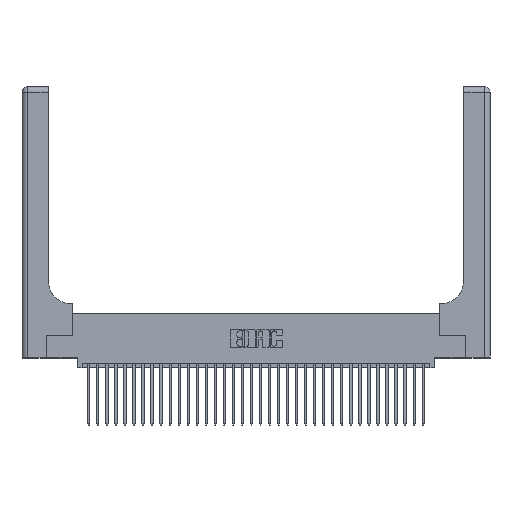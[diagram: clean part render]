
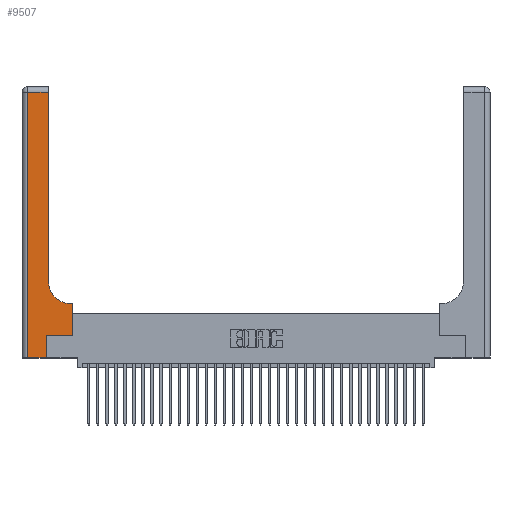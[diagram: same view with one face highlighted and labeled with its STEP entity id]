
A CAD part, top view. The second image highlights one B-rep face of the part: STEP entity #9507.
In plain terms, the highlighted planar face has unit normal (0, 0, 1).
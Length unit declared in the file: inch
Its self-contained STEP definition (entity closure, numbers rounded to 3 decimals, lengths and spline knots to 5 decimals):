
#9 = DIRECTION ( 'NONE',  ( 1., 0., 0. ) ) ;
#418 = VERTEX_POINT ( 'NONE', #31745 ) ;
#1889 = VECTOR ( 'NONE', #17187, 39.37008 ) ;
#2439 = CARTESIAN_POINT ( 'NONE',  ( 0., 0., 0.37 ) ) ;
#2482 = VECTOR ( 'NONE', #2788, 39.37008 ) ;
#2788 = DIRECTION ( 'NONE',  ( 0., 1., 0. ) ) ;
#2900 = DIRECTION ( 'NONE',  ( 0., -1., 0. ) ) ;
#3257 = CARTESIAN_POINT ( 'NONE',  ( 0.06, 3., 0.37 ) ) ;
#3908 = VERTEX_POINT ( 'NONE', #11138 ) ;
#4597 = DIRECTION ( 'NONE',  ( 0., 1., 0. ) ) ;
#4941 = EDGE_CURVE ( 'NONE', #12371, #28858, #16066, .T. ) ;
#6059 = ORIENTED_EDGE ( 'NONE', *, *, #20198, .T. ) ;
#6118 = ORIENTED_EDGE ( 'NONE', *, *, #13954, .T. ) ;
#6149 = VECTOR ( 'NONE', #17732, 39.37008 ) ;
#7418 = DIRECTION ( 'NONE',  ( 0., 0., -1. ) ) ;
#8572 = VERTEX_POINT ( 'NONE', #21850 ) ;
#9049 = VECTOR ( 'NONE', #17048, 39.37008 ) ;
#9247 = ORIENTED_EDGE ( 'NONE', *, *, #4941, .T. ) ;
#9507 = ADVANCED_FACE ( 'NONE', ( #16329 ), #17176, .F. ) ;
#9578 = LINE ( 'NONE', #3257, #25537 ) ;
#10749 = EDGE_LOOP ( 'NONE', ( #20541, #13832, #26540, #6059, #29870, #9247, #16703, #6118, #32259 ) ) ;
#11138 = CARTESIAN_POINT ( 'NONE',  ( 0.5585, 0.6, 0.37 ) ) ;
#11424 = LINE ( 'NONE', #31748, #23508 ) ;
#12316 = EDGE_CURVE ( 'NONE', #8572, #418, #11424, .T. ) ;
#12371 = VERTEX_POINT ( 'NONE', #34210 ) ;
#12557 = AXIS2_PLACEMENT_3D ( 'NONE', #22710, #7418, #23121 ) ;
#13082 = EDGE_CURVE ( 'NONE', #28672, #8572, #30018, .T. ) ;
#13832 = ORIENTED_EDGE ( 'NONE', *, *, #28359, .T. ) ;
#13954 = EDGE_CURVE ( 'NONE', #3908, #28672, #29053, .T. ) ;
#14077 = CARTESIAN_POINT ( 'NONE',  ( 0.269, 0., 0.37 ) ) ;
#14668 = DIRECTION ( 'NONE',  ( -1., 0., 0. ) ) ;
#15212 = AXIS2_PLACEMENT_3D ( 'NONE', #22901, #28441, #14668 ) ;
#16066 = LINE ( 'NONE', #30710, #6149 ) ;
#16329 = FACE_OUTER_BOUND ( 'NONE', #10749, .T. ) ;
#16703 = ORIENTED_EDGE ( 'NONE', *, *, #18743, .T. ) ;
#17048 = DIRECTION ( 'NONE',  ( 0., 1., 0. ) ) ;
#17176 = PLANE ( 'NONE',  #15212 ) ;
#17187 = DIRECTION ( 'NONE',  ( -1., 0., 0. ) ) ;
#17697 = VERTEX_POINT ( 'NONE', #33410 ) ;
#17732 = DIRECTION ( 'NONE',  ( 1., 0., 0. ) ) ;
#18025 = LINE ( 'NONE', #2439, #30174 ) ;
#18743 = EDGE_CURVE ( 'NONE', #28858, #3908, #31061, .T. ) ;
#19282 = CARTESIAN_POINT ( 'NONE',  ( 0.269, 0., 0.37 ) ) ;
#20198 = EDGE_CURVE ( 'NONE', #17697, #32036, #18025, .T. ) ;
#20541 = ORIENTED_EDGE ( 'NONE', *, *, #12316, .T. ) ;
#21850 = CARTESIAN_POINT ( 'NONE',  ( 0.2915, 0.85, 0.37 ) ) ;
#22206 = EDGE_CURVE ( 'NONE', #26370, #17697, #9578, .T. ) ;
#22268 = EDGE_CURVE ( 'NONE', #32036, #12371, #24497, .T. ) ;
#22710 = CARTESIAN_POINT ( 'NONE',  ( 0.5415, 0.85, 0.37 ) ) ;
#22901 = CARTESIAN_POINT ( 'NONE',  ( 0., 3., 0.37 ) ) ;
#23121 = DIRECTION ( 'NONE',  ( 1., 0., 0. ) ) ;
#23508 = VECTOR ( 'NONE', #4597, 39.37008 ) ;
#23515 = CARTESIAN_POINT ( 'NONE',  ( 0.5415, 0.6, 0.37 ) ) ;
#24497 = LINE ( 'NONE', #19282, #2482 ) ;
#25537 = VECTOR ( 'NONE', #2900, 39.37008 ) ;
#26370 = VERTEX_POINT ( 'NONE', #30295 ) ;
#26540 = ORIENTED_EDGE ( 'NONE', *, *, #22206, .T. ) ;
#28332 = CARTESIAN_POINT ( 'NONE',  ( 0., 2.94, 0.37 ) ) ;
#28359 = EDGE_CURVE ( 'NONE', #418, #26370, #31643, .T. ) ;
#28441 = DIRECTION ( 'NONE',  ( 0., 0., -1. ) ) ;
#28672 = VERTEX_POINT ( 'NONE', #23515 ) ;
#28858 = VERTEX_POINT ( 'NONE', #30726 ) ;
#29053 = LINE ( 'NONE', #30523, #30346 ) ;
#29870 = ORIENTED_EDGE ( 'NONE', *, *, #22268, .T. ) ;
#30018 = CIRCLE ( 'NONE', #12557, 0.25 ) ;
#30174 = VECTOR ( 'NONE', #9, 39.37008 ) ;
#30295 = CARTESIAN_POINT ( 'NONE',  ( 0.06, 2.94, 0.37 ) ) ;
#30346 = VECTOR ( 'NONE', #32852, 39.37008 ) ;
#30523 = CARTESIAN_POINT ( 'NONE',  ( 0.2915, 0.6, 0.37 ) ) ;
#30710 = CARTESIAN_POINT ( 'NONE',  ( 0.269, 0.25, 0.37 ) ) ;
#30726 = CARTESIAN_POINT ( 'NONE',  ( 0.5585, 0.25, 0.37 ) ) ;
#31061 = LINE ( 'NONE', #31483, #9049 ) ;
#31483 = CARTESIAN_POINT ( 'NONE',  ( 0.5585, 0.25, 0.37 ) ) ;
#31643 = LINE ( 'NONE', #28332, #1889 ) ;
#31745 = CARTESIAN_POINT ( 'NONE',  ( 0.2915, 2.94, 0.37 ) ) ;
#31748 = CARTESIAN_POINT ( 'NONE',  ( 0.2915, 3., 0.37 ) ) ;
#32036 = VERTEX_POINT ( 'NONE', #14077 ) ;
#32259 = ORIENTED_EDGE ( 'NONE', *, *, #13082, .T. ) ;
#32852 = DIRECTION ( 'NONE',  ( -1., 0., 0. ) ) ;
#33410 = CARTESIAN_POINT ( 'NONE',  ( 0.06, 0., 0.37 ) ) ;
#34210 = CARTESIAN_POINT ( 'NONE',  ( 0.269, 0.25, 0.37 ) ) ;
